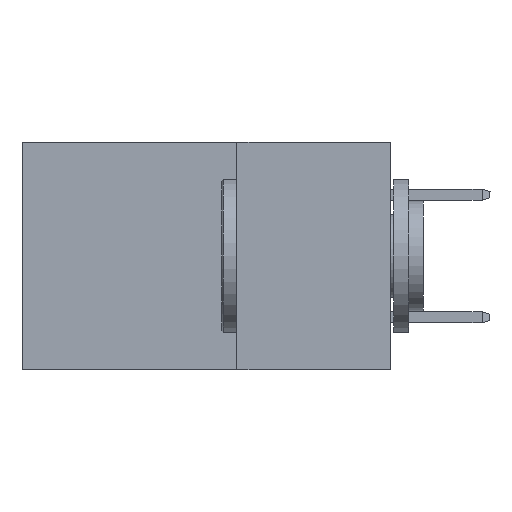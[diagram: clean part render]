
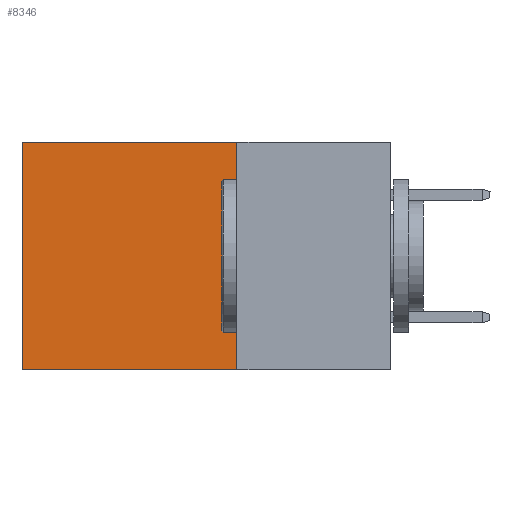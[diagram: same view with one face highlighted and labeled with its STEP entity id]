
A CAD part, left-side view. The second image highlights one B-rep face of the part: STEP entity #8346.
In plain terms, the highlighted planar face has unit normal (-1, 0, 0).
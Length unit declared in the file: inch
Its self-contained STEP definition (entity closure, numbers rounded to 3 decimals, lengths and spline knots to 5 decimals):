
#240 = CARTESIAN_POINT ( 'NONE',  ( 0.2875, 0.25, 0. ) ) ;
#694 = DIRECTION ( 'NONE',  ( 0., 1., 0. ) ) ;
#857 = EDGE_CURVE ( 'NONE', #8773, #1614, #13330, .T. ) ;
#858 = VECTOR ( 'NONE', #12720, 39.37008 ) ;
#1614 = VERTEX_POINT ( 'NONE', #11485 ) ;
#2668 = VECTOR ( 'NONE', #7960, 39.37008 ) ;
#4013 = EDGE_CURVE ( 'NONE', #8773, #7962, #6580, .T. ) ;
#4712 = DIRECTION ( 'NONE',  ( 1., 0., 0. ) ) ;
#4736 = EDGE_CURVE ( 'NONE', #1614, #14195, #10843, .T. ) ;
#4813 = EDGE_CURVE ( 'NONE', #7962, #14195, #7658, .T. ) ;
#5853 = DIRECTION ( 'NONE',  ( 0., 0., -1. ) ) ;
#6046 = VECTOR ( 'NONE', #8986, 39.37008 ) ;
#6580 = LINE ( 'NONE', #240, #858 ) ;
#6752 = ORIENTED_EDGE ( 'NONE', *, *, #4013, .F. ) ;
#6894 = ORIENTED_EDGE ( 'NONE', *, *, #4736, .T. ) ;
#7158 = CARTESIAN_POINT ( 'NONE',  ( 0.2875, 0.6, -0.37 ) ) ;
#7570 = CARTESIAN_POINT ( 'NONE',  ( 0.2875, 0.25, 0. ) ) ;
#7658 = LINE ( 'NONE', #10428, #2668 ) ;
#7960 = DIRECTION ( 'NONE',  ( 0., 1., 0. ) ) ;
#7962 = VERTEX_POINT ( 'NONE', #14052 ) ;
#8346 = ADVANCED_FACE ( 'NONE', ( #14519 ), #14808, .F. ) ;
#8683 = CARTESIAN_POINT ( 'NONE',  ( 0.2875, 0.25, 0. ) ) ;
#8773 = VERTEX_POINT ( 'NONE', #8683 ) ;
#8858 = ORIENTED_EDGE ( 'NONE', *, *, #857, .T. ) ;
#8986 = DIRECTION ( 'NONE',  ( 0., 0., -1. ) ) ;
#9227 = ORIENTED_EDGE ( 'NONE', *, *, #4813, .F. ) ;
#9903 = EDGE_LOOP ( 'NONE', ( #6894, #9227, #6752, #8858 ) ) ;
#10173 = AXIS2_PLACEMENT_3D ( 'NONE', #11478, #4712, #5853 ) ;
#10428 = CARTESIAN_POINT ( 'NONE',  ( 0.2875, 0.25, -0.37 ) ) ;
#10843 = LINE ( 'NONE', #13680, #6046 ) ;
#11478 = CARTESIAN_POINT ( 'NONE',  ( 0.2875, 0.25, 0. ) ) ;
#11485 = CARTESIAN_POINT ( 'NONE',  ( 0.2875, 0.6, 0. ) ) ;
#12720 = DIRECTION ( 'NONE',  ( 0., 0., -1. ) ) ;
#13330 = LINE ( 'NONE', #7570, #14226 ) ;
#13680 = CARTESIAN_POINT ( 'NONE',  ( 0.2875, 0.6, 0. ) ) ;
#14052 = CARTESIAN_POINT ( 'NONE',  ( 0.2875, 0.25, -0.37 ) ) ;
#14195 = VERTEX_POINT ( 'NONE', #7158 ) ;
#14226 = VECTOR ( 'NONE', #694, 39.37008 ) ;
#14519 = FACE_OUTER_BOUND ( 'NONE', #9903, .T. ) ;
#14808 = PLANE ( 'NONE',  #10173 ) ;
